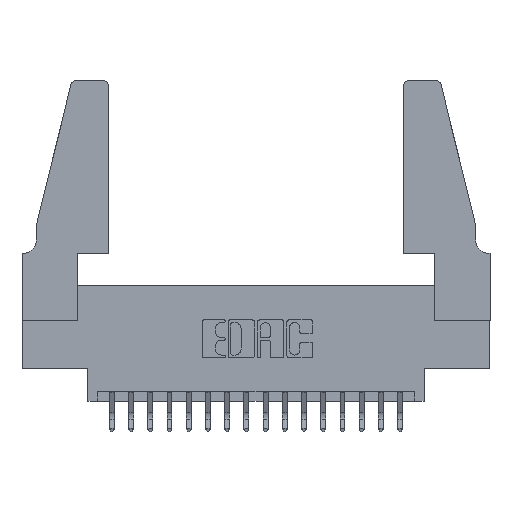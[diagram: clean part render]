
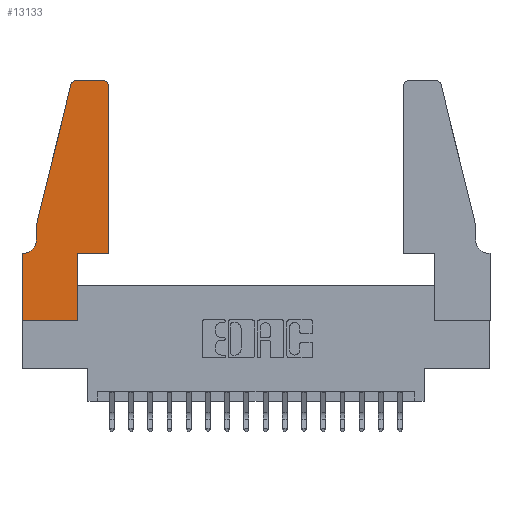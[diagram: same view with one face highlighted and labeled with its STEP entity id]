
A CAD part, top view. The second image highlights one B-rep face of the part: STEP entity #13133.
In plain terms, the highlighted planar face has unit normal (0, 0, 1).
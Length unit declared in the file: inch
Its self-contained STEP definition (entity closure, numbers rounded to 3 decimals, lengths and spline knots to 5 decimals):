
#144 = DIRECTION ( 'NONE',  ( -1., 0., 0. ) ) ;
#504 = DIRECTION ( 'NONE',  ( 1., 0., 0. ) ) ;
#562 = CIRCLE ( 'NONE', #14946, 0.03 ) ;
#722 = DIRECTION ( 'NONE',  ( 0., 0., 1. ) ) ;
#756 = CARTESIAN_POINT ( 'NONE',  ( 0.0755, 0.5, 0.37 ) ) ;
#979 = VECTOR ( 'NONE', #2233, 39.37008 ) ;
#1065 = CARTESIAN_POINT ( 'NONE',  ( 0.0055, 0.42, 0.37 ) ) ;
#1436 = FACE_OUTER_BOUND ( 'NONE', #3083, .T. ) ;
#1598 = EDGE_CURVE ( 'NONE', #18119, #3451, #13000, .T. ) ;
#1629 = EDGE_CURVE ( 'NONE', #16838, #10648, #12132, .T. ) ;
#1961 = LINE ( 'NONE', #17619, #9330 ) ;
#2069 = VECTOR ( 'NONE', #8523, 39.37008 ) ;
#2173 = DIRECTION ( 'NONE',  ( 0., 1., 0. ) ) ;
#2233 = DIRECTION ( 'NONE',  ( 0., -1., 0. ) ) ;
#2255 = CARTESIAN_POINT ( 'NONE',  ( 0.4205, 1.25, 0.37 ) ) ;
#2294 = CARTESIAN_POINT ( 'NONE',  ( 0., 0., 0.37 ) ) ;
#2539 = DIRECTION ( 'NONE',  ( -1., 0., 0. ) ) ;
#2654 = DIRECTION ( 'NONE',  ( 1., 0., 0. ) ) ;
#2782 = DIRECTION ( 'NONE',  ( 0., 0., 1. ) ) ;
#2888 = CARTESIAN_POINT ( 'NONE',  ( 0.284, 1.22, 0.37 ) ) ;
#3083 = EDGE_LOOP ( 'NONE', ( #5282, #4664, #11560, #10550, #8737, #17191, #12913, #4142, #16392, #5126, #12838, #9673 ) ) ;
#3277 = CARTESIAN_POINT ( 'NONE',  ( 0.4505, 1.22, 0.37 ) ) ;
#3383 = LINE ( 'NONE', #12439, #14413 ) ;
#3444 = CARTESIAN_POINT ( 'NONE',  ( 0.284, 1.25, 0.37 ) ) ;
#3451 = VERTEX_POINT ( 'NONE', #13336 ) ;
#3672 = VECTOR ( 'NONE', #3694, 39.37008 ) ;
#3684 = CARTESIAN_POINT ( 'NONE',  ( 0.4505, 0.35, 0.37 ) ) ;
#3694 = DIRECTION ( 'NONE',  ( 0., 1., 0. ) ) ;
#3880 = VECTOR ( 'NONE', #18587, 39.37008 ) ;
#4015 = VERTEX_POINT ( 'NONE', #5848 ) ;
#4142 = ORIENTED_EDGE ( 'NONE', *, *, #10763, .T. ) ;
#4664 = ORIENTED_EDGE ( 'NONE', *, *, #1598, .T. ) ;
#4783 = AXIS2_PLACEMENT_3D ( 'NONE', #1065, #11258, #2539 ) ;
#5126 = ORIENTED_EDGE ( 'NONE', *, *, #6569, .T. ) ;
#5237 = VERTEX_POINT ( 'NONE', #3277 ) ;
#5282 = ORIENTED_EDGE ( 'NONE', *, *, #18534, .T. ) ;
#5333 = VERTEX_POINT ( 'NONE', #9373 ) ;
#5848 = CARTESIAN_POINT ( 'NONE',  ( 0.2865, 0.35, 0.37 ) ) ;
#6070 = LINE ( 'NONE', #12694, #2069 ) ;
#6129 = EDGE_CURVE ( 'NONE', #8799, #12513, #16349, .T. ) ;
#6569 = EDGE_CURVE ( 'NONE', #4015, #15448, #1961, .T. ) ;
#6637 = EDGE_CURVE ( 'NONE', #5237, #6691, #562, .T. ) ;
#6691 = VERTEX_POINT ( 'NONE', #2255 ) ;
#7290 = CARTESIAN_POINT ( 'NONE',  ( 0., 0.35, 0.37 ) ) ;
#7651 = LINE ( 'NONE', #9516, #3672 ) ;
#7671 = LINE ( 'NONE', #3684, #10517 ) ;
#8272 = DIRECTION ( 'NONE',  ( 1., 0., 0. ) ) ;
#8298 = VECTOR ( 'NONE', #144, 39.37008 ) ;
#8523 = DIRECTION ( 'NONE',  ( -1., 0., 0. ) ) ;
#8723 = DIRECTION ( 'NONE',  ( 1., 0., 0. ) ) ;
#8737 = ORIENTED_EDGE ( 'NONE', *, *, #6129, .T. ) ;
#8799 = VERTEX_POINT ( 'NONE', #10595 ) ;
#8906 = AXIS2_PLACEMENT_3D ( 'NONE', #2888, #2782, #2654 ) ;
#9034 = CARTESIAN_POINT ( 'NONE',  ( 0.2605, 1.25, 0.37 ) ) ;
#9234 = LINE ( 'NONE', #756, #12530 ) ;
#9330 = VECTOR ( 'NONE', #504, 39.37008 ) ;
#9373 = CARTESIAN_POINT ( 'NONE',  ( 0.2865, 0., 0.37 ) ) ;
#9516 = CARTESIAN_POINT ( 'NONE',  ( 0.2865, 0.35, 0.37 ) ) ;
#9518 = CARTESIAN_POINT ( 'NONE',  ( 0.4205, 1.22, 0.37 ) ) ;
#9673 = ORIENTED_EDGE ( 'NONE', *, *, #6637, .T. ) ;
#10154 = CARTESIAN_POINT ( 'NONE',  ( 0.0055, 0.35, 0.37 ) ) ;
#10243 = EDGE_CURVE ( 'NONE', #12513, #16838, #6070, .T. ) ;
#10517 = VECTOR ( 'NONE', #2173, 39.37008 ) ;
#10550 = ORIENTED_EDGE ( 'NONE', *, *, #14678, .T. ) ;
#10595 = CARTESIAN_POINT ( 'NONE',  ( 0.0755, 0.42, 0.37 ) ) ;
#10648 = VERTEX_POINT ( 'NONE', #17747 ) ;
#10763 = EDGE_CURVE ( 'NONE', #10648, #5333, #3383, .T. ) ;
#10937 = DIRECTION ( 'NONE',  ( 1., 0., 0. ) ) ;
#11258 = DIRECTION ( 'NONE',  ( 0., 0., -1. ) ) ;
#11560 = ORIENTED_EDGE ( 'NONE', *, *, #17916, .T. ) ;
#12048 = CARTESIAN_POINT ( 'NONE',  ( 0., 0.35, 0.37 ) ) ;
#12132 = LINE ( 'NONE', #2294, #979 ) ;
#12344 = CARTESIAN_POINT ( 'NONE',  ( 0.0755, 0.5, 0.37 ) ) ;
#12439 = CARTESIAN_POINT ( 'NONE',  ( 0., 0., 0.37 ) ) ;
#12513 = VERTEX_POINT ( 'NONE', #10154 ) ;
#12530 = VECTOR ( 'NONE', #13796, 39.37008 ) ;
#12694 = CARTESIAN_POINT ( 'NONE',  ( 0.0755, 0.35, 0.37 ) ) ;
#12838 = ORIENTED_EDGE ( 'NONE', *, *, #16962, .T. ) ;
#12887 = LINE ( 'NONE', #9034, #8298 ) ;
#12913 = ORIENTED_EDGE ( 'NONE', *, *, #1629, .T. ) ;
#13000 = CIRCLE ( 'NONE', #8906, 0.03 ) ;
#13133 = ADVANCED_FACE ( 'NONE', ( #1436 ), #15694, .T. ) ;
#13336 = CARTESIAN_POINT ( 'NONE',  ( 0.25487, 1.22718, 0.37 ) ) ;
#13796 = DIRECTION ( 'NONE',  ( 0., -1., 0. ) ) ;
#14413 = VECTOR ( 'NONE', #8272, 39.37008 ) ;
#14678 = EDGE_CURVE ( 'NONE', #16954, #8799, #9234, .T. ) ;
#14946 = AXIS2_PLACEMENT_3D ( 'NONE', #9518, #722, #10937 ) ;
#14948 = AXIS2_PLACEMENT_3D ( 'NONE', #7290, #17082, #8723 ) ;
#15300 = LINE ( 'NONE', #17221, #3880 ) ;
#15448 = VERTEX_POINT ( 'NONE', #18087 ) ;
#15694 = PLANE ( 'NONE',  #14948 ) ;
#15849 = EDGE_CURVE ( 'NONE', #5333, #4015, #7651, .T. ) ;
#16349 = CIRCLE ( 'NONE', #4783, 0.07 ) ;
#16392 = ORIENTED_EDGE ( 'NONE', *, *, #15849, .T. ) ;
#16838 = VERTEX_POINT ( 'NONE', #12048 ) ;
#16954 = VERTEX_POINT ( 'NONE', #12344 ) ;
#16962 = EDGE_CURVE ( 'NONE', #15448, #5237, #7671, .T. ) ;
#17082 = DIRECTION ( 'NONE',  ( 0., 0., 1. ) ) ;
#17191 = ORIENTED_EDGE ( 'NONE', *, *, #10243, .T. ) ;
#17221 = CARTESIAN_POINT ( 'NONE',  ( 0.0755, 0.5, 0.37 ) ) ;
#17619 = CARTESIAN_POINT ( 'NONE',  ( 0.4505, 0.35, 0.37 ) ) ;
#17747 = CARTESIAN_POINT ( 'NONE',  ( 0., 0., 0.37 ) ) ;
#17916 = EDGE_CURVE ( 'NONE', #3451, #16954, #15300, .T. ) ;
#18087 = CARTESIAN_POINT ( 'NONE',  ( 0.4505, 0.35, 0.37 ) ) ;
#18119 = VERTEX_POINT ( 'NONE', #3444 ) ;
#18534 = EDGE_CURVE ( 'NONE', #6691, #18119, #12887, .T. ) ;
#18587 = DIRECTION ( 'NONE',  ( -0.239, -0.971, 0. ) ) ;
